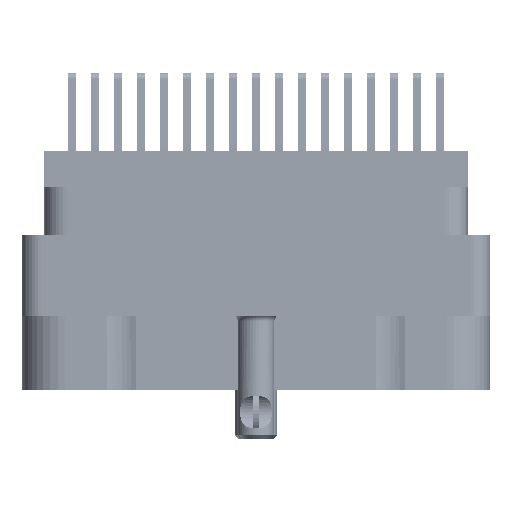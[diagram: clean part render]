
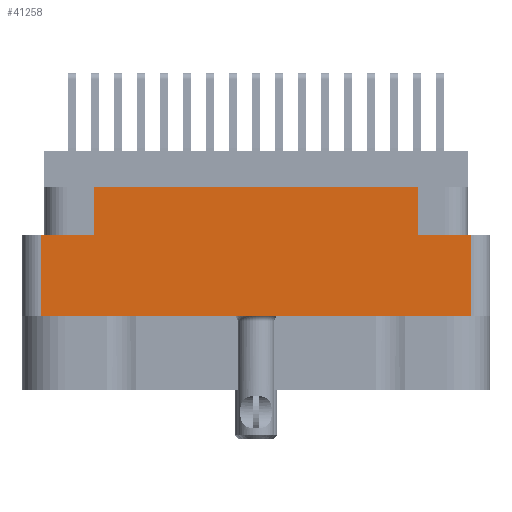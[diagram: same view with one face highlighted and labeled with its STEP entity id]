
A CAD part, left-side view. The second image highlights one B-rep face of the part: STEP entity #41258.
In plain terms, the highlighted planar face has unit normal (-1, 0, 0).
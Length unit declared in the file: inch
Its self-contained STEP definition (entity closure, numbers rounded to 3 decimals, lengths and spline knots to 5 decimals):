
#1446 = EDGE_LOOP ( 'NONE', ( #89910, #11854, #82347, #8185, #27219, #72399, #56730, #94091 ) ) ;
#3510 = CARTESIAN_POINT ( 'NONE',  ( -1.375, 0.5285, -0.274 ) ) ;
#5663 = LINE ( 'NONE', #84044, #89579 ) ;
#5702 = DIRECTION ( 'NONE',  ( 0., -1., 0. ) ) ;
#8185 = ORIENTED_EDGE ( 'NONE', *, *, #23889, .T. ) ;
#9665 = LINE ( 'NONE', #3510, #31966 ) ;
#11854 = ORIENTED_EDGE ( 'NONE', *, *, #96771, .T. ) ;
#17226 = AXIS2_PLACEMENT_3D ( 'NONE', #22630, #99966, #60303 ) ;
#20981 = LINE ( 'NONE', #75486, #68879 ) ;
#22423 = VERTEX_POINT ( 'NONE', #34715 ) ;
#22630 = CARTESIAN_POINT ( 'NONE',  ( -1.375, -0.7625, -0.78 ) ) ;
#23889 = EDGE_CURVE ( 'NONE', #72050, #79724, #52492, .T. ) ;
#24536 = LINE ( 'NONE', #76493, #62537 ) ;
#27219 = ORIENTED_EDGE ( 'NONE', *, *, #38400, .F. ) ;
#30083 = DIRECTION ( 'NONE',  ( 0., 0., 1. ) ) ;
#31966 = VECTOR ( 'NONE', #65675, 39.37008 ) ;
#32214 = LINE ( 'NONE', #63315, #90376 ) ;
#34715 = CARTESIAN_POINT ( 'NONE',  ( -1.375, 0.5285, -0.117 ) ) ;
#35288 = EDGE_CURVE ( 'NONE', #22423, #95080, #99038, .T. ) ;
#35874 = VECTOR ( 'NONE', #45608, 39.37008 ) ;
#36148 = CARTESIAN_POINT ( 'NONE',  ( -1.375, 0., -0.274 ) ) ;
#37194 = DIRECTION ( 'NONE',  ( 0., 0., 1. ) ) ;
#38400 = EDGE_CURVE ( 'NONE', #93275, #79724, #20981, .T. ) ;
#41086 = VECTOR ( 'NONE', #67225, 39.37008 ) ;
#41258 = ADVANCED_FACE ( 'NONE', ( #68987 ), #53682, .T. ) ;
#41975 = CARTESIAN_POINT ( 'NONE',  ( -1.375, -0.5285, -0.117 ) ) ;
#45108 = CARTESIAN_POINT ( 'NONE',  ( -1.375, -0.5285, -0.274 ) ) ;
#45140 = CARTESIAN_POINT ( 'NONE',  ( -1.375, -0.7005, -0.54 ) ) ;
#45608 = DIRECTION ( 'NONE',  ( 0., -1., 0. ) ) ;
#48080 = VECTOR ( 'NONE', #37194, 39.37008 ) ;
#49142 = EDGE_CURVE ( 'NONE', #99476, #72050, #24536, .T. ) ;
#50374 = VERTEX_POINT ( 'NONE', #73656 ) ;
#51090 = EDGE_CURVE ( 'NONE', #50374, #22423, #9665, .T. ) ;
#51620 = CARTESIAN_POINT ( 'NONE',  ( -1.375, 0.7005, -0.54 ) ) ;
#52492 = LINE ( 'NONE', #75921, #48080 ) ;
#53571 = DIRECTION ( 'NONE',  ( 0., -1., 0. ) ) ;
#53682 = PLANE ( 'NONE',  #17226 ) ;
#54644 = DIRECTION ( 'NONE',  ( 0., 0., -1. ) ) ;
#56730 = ORIENTED_EDGE ( 'NONE', *, *, #35288, .F. ) ;
#58185 = EDGE_CURVE ( 'NONE', #93275, #95080, #5663, .T. ) ;
#60303 = DIRECTION ( 'NONE',  ( 0., 0., 1. ) ) ;
#62537 = VECTOR ( 'NONE', #53571, 39.37008 ) ;
#63315 = CARTESIAN_POINT ( 'NONE',  ( -1.375, 0.7005, -0.78 ) ) ;
#65236 = LINE ( 'NONE', #36148, #41086 ) ;
#65675 = DIRECTION ( 'NONE',  ( 0., 0., 1. ) ) ;
#67225 = DIRECTION ( 'NONE',  ( 0., -1., 0. ) ) ;
#67552 = CARTESIAN_POINT ( 'NONE',  ( -1.375, 0.7625, -0.117 ) ) ;
#68879 = VECTOR ( 'NONE', #5702, 39.37008 ) ;
#68987 = FACE_OUTER_BOUND ( 'NONE', #1446, .T. ) ;
#69453 = VERTEX_POINT ( 'NONE', #89009 ) ;
#72050 = VERTEX_POINT ( 'NONE', #45140 ) ;
#72399 = ORIENTED_EDGE ( 'NONE', *, *, #58185, .T. ) ;
#73656 = CARTESIAN_POINT ( 'NONE',  ( -1.375, 0.5285, -0.274 ) ) ;
#75486 = CARTESIAN_POINT ( 'NONE',  ( -1.375, 0., -0.274 ) ) ;
#75921 = CARTESIAN_POINT ( 'NONE',  ( -1.375, -0.7005, -0.78 ) ) ;
#76493 = CARTESIAN_POINT ( 'NONE',  ( -1.375, 0., -0.54 ) ) ;
#79724 = VERTEX_POINT ( 'NONE', #99724 ) ;
#82347 = ORIENTED_EDGE ( 'NONE', *, *, #49142, .T. ) ;
#84044 = CARTESIAN_POINT ( 'NONE',  ( -1.375, -0.5285, -0.274 ) ) ;
#86564 = EDGE_CURVE ( 'NONE', #69453, #50374, #65236, .T. ) ;
#89009 = CARTESIAN_POINT ( 'NONE',  ( -1.375, 0.7005, -0.274 ) ) ;
#89579 = VECTOR ( 'NONE', #30083, 39.37008 ) ;
#89910 = ORIENTED_EDGE ( 'NONE', *, *, #86564, .F. ) ;
#90376 = VECTOR ( 'NONE', #54644, 39.37008 ) ;
#93275 = VERTEX_POINT ( 'NONE', #45108 ) ;
#94091 = ORIENTED_EDGE ( 'NONE', *, *, #51090, .F. ) ;
#95080 = VERTEX_POINT ( 'NONE', #41975 ) ;
#96771 = EDGE_CURVE ( 'NONE', #69453, #99476, #32214, .T. ) ;
#99038 = LINE ( 'NONE', #67552, #35874 ) ;
#99476 = VERTEX_POINT ( 'NONE', #51620 ) ;
#99724 = CARTESIAN_POINT ( 'NONE',  ( -1.375, -0.7005, -0.274 ) ) ;
#99966 = DIRECTION ( 'NONE',  ( -1., 0., 0. ) ) ;
